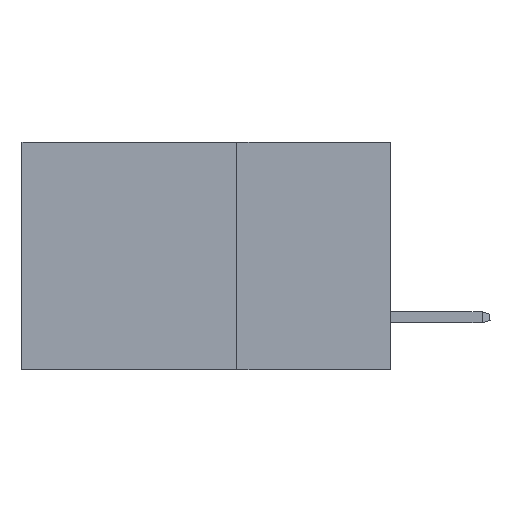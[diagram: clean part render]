
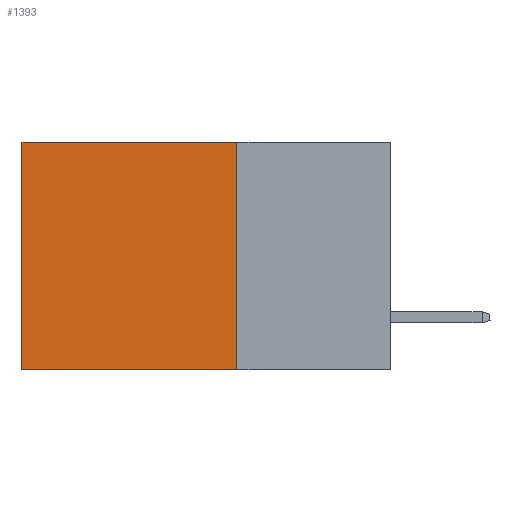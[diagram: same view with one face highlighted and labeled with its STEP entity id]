
A CAD part, left-side view. The second image highlights one B-rep face of the part: STEP entity #1393.
In plain terms, the highlighted planar face has unit normal (-1, 0, 0).
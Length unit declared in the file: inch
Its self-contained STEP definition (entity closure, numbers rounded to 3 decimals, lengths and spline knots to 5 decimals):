
#1200 = EDGE_CURVE ( 'NONE', #18213, #5842, #21779, .T. ) ;
#1317 = VECTOR ( 'NONE', #6396, 39.37008 ) ;
#1393 = ADVANCED_FACE ( 'NONE', ( #4201 ), #11883, .F. ) ;
#1450 = VERTEX_POINT ( 'NONE', #7992 ) ;
#1757 = EDGE_CURVE ( 'NONE', #10247, #1450, #13289, .T. ) ;
#2227 = ORIENTED_EDGE ( 'NONE', *, *, #12143, .T. ) ;
#4201 = FACE_OUTER_BOUND ( 'NONE', #16783, .T. ) ;
#4315 = CARTESIAN_POINT ( 'NONE',  ( 0.2875, 0.25, 0. ) ) ;
#4997 = DIRECTION ( 'NONE',  ( 0., 0., -1. ) ) ;
#5842 = VERTEX_POINT ( 'NONE', #12430 ) ;
#6396 = DIRECTION ( 'NONE',  ( 0., 0., -1. ) ) ;
#6481 = VECTOR ( 'NONE', #17064, 39.37008 ) ;
#7992 = CARTESIAN_POINT ( 'NONE',  ( 0.2875, 0.6, -0.37 ) ) ;
#10247 = VERTEX_POINT ( 'NONE', #17098 ) ;
#10312 = ORIENTED_EDGE ( 'NONE', *, *, #1757, .T. ) ;
#10573 = VECTOR ( 'NONE', #21194, 39.37008 ) ;
#11883 = PLANE ( 'NONE',  #23617 ) ;
#12143 = EDGE_CURVE ( 'NONE', #18213, #10247, #24023, .T. ) ;
#12430 = CARTESIAN_POINT ( 'NONE',  ( 0.2875, 0.25, -0.37 ) ) ;
#13289 = LINE ( 'NONE', #20986, #13872 ) ;
#13872 = VECTOR ( 'NONE', #4997, 39.37008 ) ;
#13958 = CARTESIAN_POINT ( 'NONE',  ( 0.2875, 0.25, -0.37 ) ) ;
#15330 = DIRECTION ( 'NONE',  ( 1., 0., 0. ) ) ;
#15540 = LINE ( 'NONE', #13958, #10573 ) ;
#16783 = EDGE_LOOP ( 'NONE', ( #10312, #18467, #23012, #2227 ) ) ;
#16987 = CARTESIAN_POINT ( 'NONE',  ( 0.2875, 0.25, 0. ) ) ;
#17064 = DIRECTION ( 'NONE',  ( 0., 1., 0. ) ) ;
#17098 = CARTESIAN_POINT ( 'NONE',  ( 0.2875, 0.6, 0. ) ) ;
#17449 = CARTESIAN_POINT ( 'NONE',  ( 0.2875, 0.25, 0. ) ) ;
#18213 = VERTEX_POINT ( 'NONE', #21248 ) ;
#18467 = ORIENTED_EDGE ( 'NONE', *, *, #21418, .F. ) ;
#20986 = CARTESIAN_POINT ( 'NONE',  ( 0.2875, 0.6, 0. ) ) ;
#21194 = DIRECTION ( 'NONE',  ( 0., 1., 0. ) ) ;
#21248 = CARTESIAN_POINT ( 'NONE',  ( 0.2875, 0.25, 0. ) ) ;
#21418 = EDGE_CURVE ( 'NONE', #5842, #1450, #15540, .T. ) ;
#21779 = LINE ( 'NONE', #4315, #1317 ) ;
#22920 = DIRECTION ( 'NONE',  ( 0., 0., -1. ) ) ;
#23012 = ORIENTED_EDGE ( 'NONE', *, *, #1200, .F. ) ;
#23617 = AXIS2_PLACEMENT_3D ( 'NONE', #17449, #15330, #22920 ) ;
#24023 = LINE ( 'NONE', #16987, #6481 ) ;
